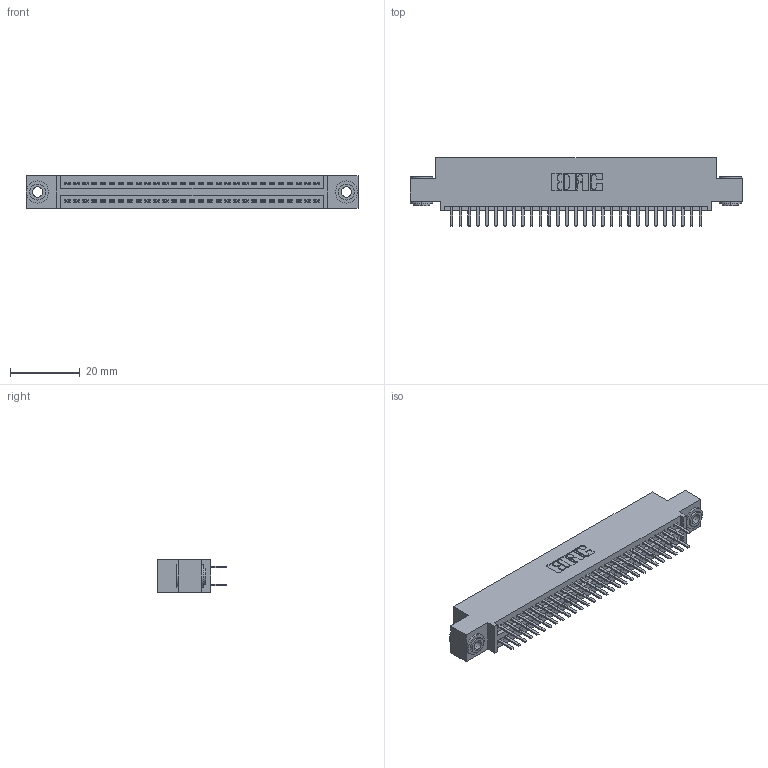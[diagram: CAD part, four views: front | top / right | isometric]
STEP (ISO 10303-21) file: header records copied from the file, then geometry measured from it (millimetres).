
FILE_DESCRIPTION (( 'STEP AP203' ), '1' );
FILE_NAME ('345-058-520-503.STEP', '2019-10-30T04:24:49', ( '' ), ( '' ), 'SwSTEP 2.0', 'SolidWorks 2016', '' );
FILE_SCHEMA (( 'CONFIG_CONTROL_DESIGN' ));
Length unit declared in the file: inch
Products named in the file (4): 345-250-002_345-250-002-102; 345-292-001_345-293-120; 345-058-520-503; 345 Part_0.110 Offset - 0.156 Dia-TH
Assembly tree (61 placements, depth 2):
  345-058-520-503
    345 Part_0.110 Offset - 0.156 Dia-TH
    345-292-001_345-293-120  x58
    345-250-002_345-250-002-102  x2
Bounding box: 94.87 x 19.68 x 9.4 mm (x, y, z)
Volume: 9015.5 mm3; surface area: 13318.2 mm2
Topology: 61 solids, 61 shells, 3300 faces, 9535 edges, 6198 vertices
Faces by surface type: plane 2124, cylinder 1168, cone 8
Entity records: 25400 total; most frequent: CARTESIAN_POINT 4259, ORIENTED_EDGE 4174, DIRECTION 3789, EDGE_CURVE 2087, LINE 1811, VECTOR 1811, VERTEX_POINT 1386, AXIS2_PLACEMENT_3D 989
